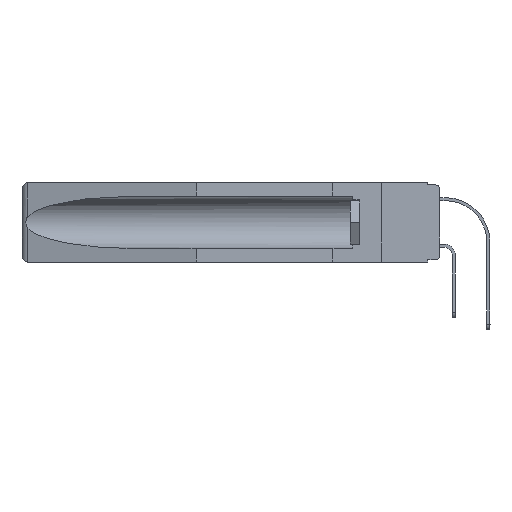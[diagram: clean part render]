
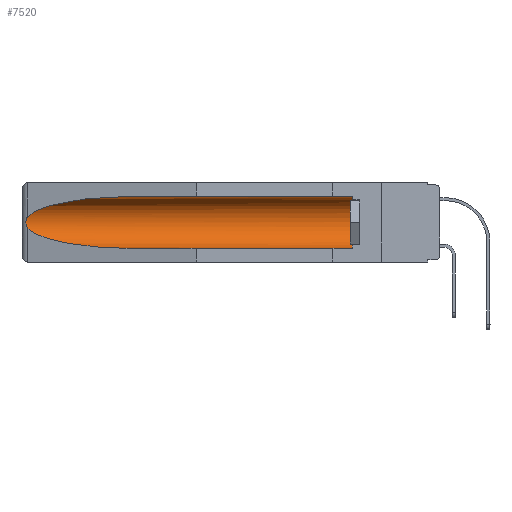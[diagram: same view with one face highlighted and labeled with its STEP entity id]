
A CAD part, left-side view. The second image highlights one B-rep face of the part: STEP entity #7520.
In plain terms, the highlighted cylindrical face has radius 2.857 mm (diameter 5.715 mm), a partial arc.
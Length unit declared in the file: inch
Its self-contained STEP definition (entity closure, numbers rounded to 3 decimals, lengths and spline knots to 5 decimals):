
#301 = B_SPLINE_CURVE_WITH_KNOTS ( 'NONE', 3,
 ( #10549, #2600, #15152, #7530, #8729, #1502, #1203, #13660, #13254, #14853 ),
 .UNSPECIFIED., .F., .F.,
 ( 4, 2, 2, 2, 4 ),
 ( 0., 0.00029, 0.00058, 0.00087, 0.00117 ),
 .UNSPECIFIED. ) ;
#775 = CARTESIAN_POINT ( 'NONE',  ( 0.155, 1.07973, -0.284 ) ) ;
#1203 = CARTESIAN_POINT ( 'NONE',  ( 0.2673, 1.53269, -0.17917 ) ) ;
#1502 = CARTESIAN_POINT ( 'NONE',  ( 0.2675, 1.53308, -0.17534 ) ) ;
#1693 = VERTEX_POINT ( 'NONE', #11092 ) ;
#2001 = EDGE_CURVE ( 'NONE', #1693, #11089, #12912, .T. ) ;
#2600 = CARTESIAN_POINT ( 'NONE',  ( 0.26597, 1.52961, -0.15275 ) ) ;
#2613 = CIRCLE ( 'NONE', #6468, 0.1125 ) ;
#2718 = CARTESIAN_POINT ( 'NONE',  ( 0.26537, 1.52718, -0.14972 ) ) ;
#2729 = DIRECTION ( 'NONE',  ( 0., 1., 0. ) ) ;
#3147 = CARTESIAN_POINT ( 'NONE',  ( 0.26537, 1.52718, -0.19328 ) ) ;
#3177 =( BOUNDED_CURVE ( )  B_SPLINE_CURVE ( 3, ( #5841, #16466, #18078, #2718 ),
 .UNSPECIFIED., .F., .F. ) 
 B_SPLINE_CURVE_WITH_KNOTS ( ( 4, 4 ),
 ( 4.71239, 6.08839 ),
 .UNSPECIFIED. ) 
 CURVE ( )  GEOMETRIC_REPRESENTATION_ITEM ( )  RATIONAL_B_SPLINE_CURVE ( ( 1., 0.848, 0.848, 1. ) ) 
 REPRESENTATION_ITEM ( '' )  );
#3418 = CARTESIAN_POINT ( 'NONE',  ( 0.26537, 1.52718, -0.14972 ) ) ;
#3933 = VERTEX_POINT ( 'NONE', #3418 ) ;
#4447 = CYLINDRICAL_SURFACE ( 'NONE', #16927, 0.1125 ) ;
#4454 = CARTESIAN_POINT ( 'NONE',  ( 0.155, 1.07973, -0.284 ) ) ;
#4540 = FACE_OUTER_BOUND ( 'NONE', #7611, .T. ) ;
#4649 = CARTESIAN_POINT ( 'NONE',  ( 0.155, 0.126, -0.059 ) ) ;
#5259 = VECTOR ( 'NONE', #18539, 39.37008 ) ;
#5660 = ORIENTED_EDGE ( 'NONE', *, *, #8578, .F. ) ;
#5761 = ORIENTED_EDGE ( 'NONE', *, *, #2001, .T. ) ;
#5841 = CARTESIAN_POINT ( 'NONE',  ( 0.155, 1.07973, -0.059 ) ) ;
#6468 = AXIS2_PLACEMENT_3D ( 'NONE', #7533, #18273, #10746 ) ;
#6815 = VERTEX_POINT ( 'NONE', #17151 ) ;
#6894 = LINE ( 'NONE', #17332, #11723 ) ;
#6990 = DIRECTION ( 'NONE',  ( 0., 1., 0. ) ) ;
#7251 = DIRECTION ( 'NONE',  ( 0., 0., 1. ) ) ;
#7313 = ORIENTED_EDGE ( 'NONE', *, *, #16010, .T. ) ;
#7520 = ADVANCED_FACE ( 'NONE', ( #4540 ), #4447, .F. ) ;
#7530 = CARTESIAN_POINT ( 'NONE',  ( 0.2673, 1.5327, -0.16383 ) ) ;
#7533 = CARTESIAN_POINT ( 'NONE',  ( 0.155, 0.126, -0.1715 ) ) ;
#7611 = EDGE_LOOP ( 'NONE', ( #10283, #19212, #5761, #5660, #16327, #7313 ) ) ;
#7696 = CARTESIAN_POINT ( 'NONE',  ( 0.155, -0.30754, -0.284 ) ) ;
#8033 = EDGE_CURVE ( 'NONE', #3933, #1693, #301, .T. ) ;
#8578 = EDGE_CURVE ( 'NONE', #19674, #11089, #10609, .T. ) ;
#8729 = CARTESIAN_POINT ( 'NONE',  ( 0.2675, 1.53308, -0.16763 ) ) ;
#9236 = CARTESIAN_POINT ( 'NONE',  ( 0.155, 0.126, -0.284 ) ) ;
#9264 = CARTESIAN_POINT ( 'NONE',  ( 0.25451, 1.48313, -0.24835 ) ) ;
#10283 = ORIENTED_EDGE ( 'NONE', *, *, #15419, .T. ) ;
#10549 = CARTESIAN_POINT ( 'NONE',  ( 0.26537, 1.52718, -0.14972 ) ) ;
#10609 = LINE ( 'NONE', #7696, #5259 ) ;
#10746 = DIRECTION ( 'NONE',  ( 0., 0., 1. ) ) ;
#11089 = VERTEX_POINT ( 'NONE', #775 ) ;
#11092 = CARTESIAN_POINT ( 'NONE',  ( 0.26537, 1.52718, -0.19328 ) ) ;
#11723 = VECTOR ( 'NONE', #6990, 39.37008 ) ;
#12389 = CARTESIAN_POINT ( 'NONE',  ( 0.21114, 1.30732, -0.284 ) ) ;
#12912 =( BOUNDED_CURVE ( )  B_SPLINE_CURVE ( 3, ( #3147, #9264, #12389, #4454 ),
 .UNSPECIFIED., .F., .F. ) 
 B_SPLINE_CURVE_WITH_KNOTS ( ( 4, 4 ),
 ( 0.1948, 1.5708 ),
 .UNSPECIFIED. ) 
 CURVE ( )  GEOMETRIC_REPRESENTATION_ITEM ( )  RATIONAL_B_SPLINE_CURVE ( ( 1., 0.848, 0.848, 1. ) ) 
 REPRESENTATION_ITEM ( '' )  );
#13254 = CARTESIAN_POINT ( 'NONE',  ( 0.26597, 1.5296, -0.19026 ) ) ;
#13660 = CARTESIAN_POINT ( 'NONE',  ( 0.26655, 1.53094, -0.18657 ) ) ;
#14853 = CARTESIAN_POINT ( 'NONE',  ( 0.26537, 1.52718, -0.19328 ) ) ;
#14959 = VERTEX_POINT ( 'NONE', #4649 ) ;
#15072 = CARTESIAN_POINT ( 'NONE',  ( 0.155, -0.30754, -0.1715 ) ) ;
#15152 = CARTESIAN_POINT ( 'NONE',  ( 0.26654, 1.53092, -0.15636 ) ) ;
#15419 = EDGE_CURVE ( 'NONE', #6815, #3933, #3177, .T. ) ;
#16010 = EDGE_CURVE ( 'NONE', #14959, #6815, #6894, .T. ) ;
#16327 = ORIENTED_EDGE ( 'NONE', *, *, #19613, .T. ) ;
#16466 = CARTESIAN_POINT ( 'NONE',  ( 0.21114, 1.30732, -0.059 ) ) ;
#16927 = AXIS2_PLACEMENT_3D ( 'NONE', #15072, #2729, #7251 ) ;
#17151 = CARTESIAN_POINT ( 'NONE',  ( 0.155, 1.07973, -0.059 ) ) ;
#17332 = CARTESIAN_POINT ( 'NONE',  ( 0.155, -0.30754, -0.059 ) ) ;
#18078 = CARTESIAN_POINT ( 'NONE',  ( 0.25451, 1.48313, -0.09465 ) ) ;
#18273 = DIRECTION ( 'NONE',  ( 0., -1., 0. ) ) ;
#18539 = DIRECTION ( 'NONE',  ( 0., 1., 0. ) ) ;
#19212 = ORIENTED_EDGE ( 'NONE', *, *, #8033, .T. ) ;
#19613 = EDGE_CURVE ( 'NONE', #19674, #14959, #2613, .T. ) ;
#19674 = VERTEX_POINT ( 'NONE', #9236 ) ;
